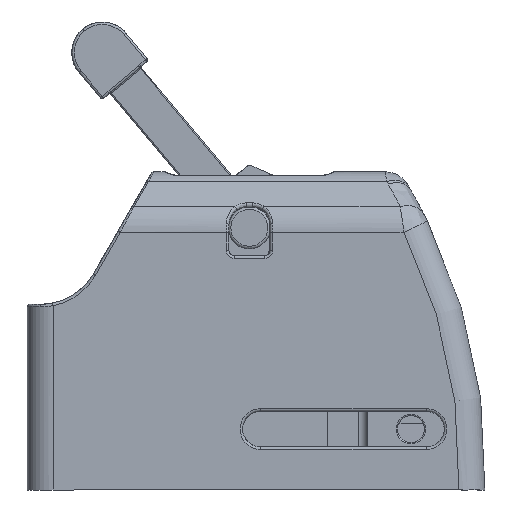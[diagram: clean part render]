
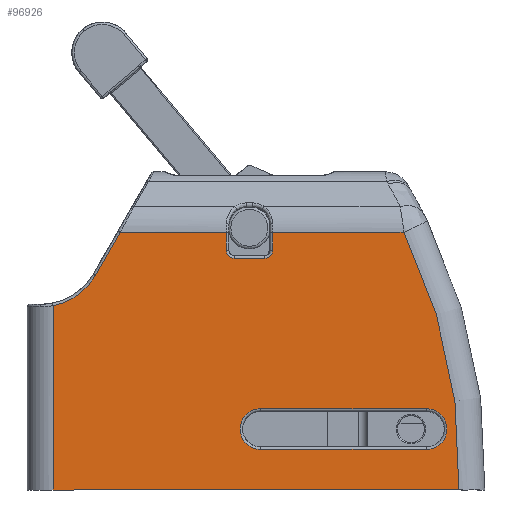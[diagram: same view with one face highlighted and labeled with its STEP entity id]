
A CAD part, left-side view. The second image highlights one B-rep face of the part: STEP entity #96926.
In plain terms, the highlighted planar face has unit normal (-1, 0, 0).
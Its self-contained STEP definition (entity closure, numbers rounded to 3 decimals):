
#5183=FACE_BOUND('',#18355,.T.);
#10724=PLANE('',#102975);
#12639=FACE_OUTER_BOUND('',#18354,.T.);
#18354=EDGE_LOOP('',(#66853,#66854,#66855,#66856,#66857,#66858,#66859,#66860,
#66861,#66862,#66863,#66864));
#18355=EDGE_LOOP('',(#66865,#66866,#66867,#66868));
#24453=LINE('',#128209,#31657);
#24456=LINE('',#128224,#31660);
#24464=LINE('',#128274,#31668);
#24465=LINE('',#128278,#31669);
#24466=LINE('',#128280,#31670);
#24467=LINE('',#128284,#31671);
#24468=LINE('',#128286,#31672);
#24469=LINE('',#128290,#31673);
#24470=LINE('',#128294,#31674);
#24471=LINE('',#128295,#31675);
#31657=VECTOR('',#108685,10.);
#31660=VECTOR('',#108702,10.);
#31668=VECTOR('',#108730,10.);
#31669=VECTOR('',#108733,10.);
#31670=VECTOR('',#108734,10.);
#31671=VECTOR('',#108737,10.);
#31672=VECTOR('',#108738,10.);
#31673=VECTOR('',#108741,10.);
#31674=VECTOR('',#108744,10.);
#31675=VECTOR('',#108745,10.);
#38824=CIRCLE('',#102963,3.925);
#38827=CIRCLE('',#102968,3.925);
#38832=CIRCLE('',#102976,12.);
#38833=CIRCLE('',#102977,103.5);
#38834=CIRCLE('',#102978,1.5);
#38835=CIRCLE('',#102979,1.5);
#40448=VERTEX_POINT('',#128206);
#40449=VERTEX_POINT('',#128208);
#40451=VERTEX_POINT('',#128214);
#40453=VERTEX_POINT('',#128220);
#40465=VERTEX_POINT('',#128272);
#40466=VERTEX_POINT('',#128273);
#40467=VERTEX_POINT('',#128275);
#40468=VERTEX_POINT('',#128277);
#40469=VERTEX_POINT('',#128279);
#40470=VERTEX_POINT('',#128281);
#40471=VERTEX_POINT('',#128283);
#40472=VERTEX_POINT('',#128285);
#40473=VERTEX_POINT('',#128287);
#40474=VERTEX_POINT('',#128289);
#40475=VERTEX_POINT('',#128291);
#40476=VERTEX_POINT('',#128293);
#50762=EDGE_CURVE('',#40448,#40449,#24453,.T.);
#50767=EDGE_CURVE('',#40449,#40451,#38824,.T.);
#50770=EDGE_CURVE('',#40451,#40453,#24456,.T.);
#50772=EDGE_CURVE('',#40453,#40448,#38827,.T.);
#50786=EDGE_CURVE('',#40465,#40466,#24464,.T.);
#50787=EDGE_CURVE('',#40467,#40465,#38832,.T.);
#50788=EDGE_CURVE('',#40468,#40467,#24465,.T.);
#50789=EDGE_CURVE('',#40468,#40469,#24466,.F.);
#50790=EDGE_CURVE('',#40470,#40469,#38833,.T.);
#50791=EDGE_CURVE('',#40470,#40471,#24467,.T.);
#50792=EDGE_CURVE('',#40472,#40471,#24468,.T.);
#50793=EDGE_CURVE('',#40473,#40472,#38834,.T.);
#50794=EDGE_CURVE('',#40474,#40473,#24469,.T.);
#50795=EDGE_CURVE('',#40475,#40474,#38835,.T.);
#50796=EDGE_CURVE('',#40476,#40475,#24470,.T.);
#50797=EDGE_CURVE('',#40476,#40466,#24471,.T.);
#66853=ORIENTED_EDGE('',*,*,#50786,.F.);
#66854=ORIENTED_EDGE('',*,*,#50787,.F.);
#66855=ORIENTED_EDGE('',*,*,#50788,.F.);
#66856=ORIENTED_EDGE('',*,*,#50789,.T.);
#66857=ORIENTED_EDGE('',*,*,#50790,.F.);
#66858=ORIENTED_EDGE('',*,*,#50791,.T.);
#66859=ORIENTED_EDGE('',*,*,#50792,.F.);
#66860=ORIENTED_EDGE('',*,*,#50793,.F.);
#66861=ORIENTED_EDGE('',*,*,#50794,.F.);
#66862=ORIENTED_EDGE('',*,*,#50795,.F.);
#66863=ORIENTED_EDGE('',*,*,#50796,.F.);
#66864=ORIENTED_EDGE('',*,*,#50797,.T.);
#66865=ORIENTED_EDGE('',*,*,#50762,.F.);
#66866=ORIENTED_EDGE('',*,*,#50772,.F.);
#66867=ORIENTED_EDGE('',*,*,#50770,.F.);
#66868=ORIENTED_EDGE('',*,*,#50767,.F.);
#96926=ADVANCED_FACE('',(#12639,#5183),#10724,.F.);
#102963=AXIS2_PLACEMENT_3D('',#128218,#108695,#108696);
#102968=AXIS2_PLACEMENT_3D('',#128227,#108707,#108708);
#102975=AXIS2_PLACEMENT_3D('',#128271,#108728,#108729);
#102976=AXIS2_PLACEMENT_3D('',#128276,#108731,#108732);
#102977=AXIS2_PLACEMENT_3D('',#128282,#108735,#108736);
#102978=AXIS2_PLACEMENT_3D('',#128288,#108739,#108740);
#102979=AXIS2_PLACEMENT_3D('',#128292,#108742,#108743);
#108685=DIRECTION('',(0.,-1.,0.));
#108695=DIRECTION('center_axis',(-1.,0.,0.));
#108696=DIRECTION('ref_axis',(0.,-1.,0.));
#108702=DIRECTION('',(0.,1.,0.));
#108707=DIRECTION('center_axis',(-1.,0.,0.));
#108708=DIRECTION('ref_axis',(0.,1.,0.));
#108728=DIRECTION('center_axis',(1.,0.,0.));
#108729=DIRECTION('ref_axis',(0.,0.,-1.));
#108730=DIRECTION('',(0.,-0.499,0.866));
#108731=DIRECTION('center_axis',(-1.,0.,0.));
#108732=DIRECTION('ref_axis',(0.,-0.583,-0.812));
#108733=DIRECTION('',(0.,0.,1.));
#108734=DIRECTION('',(0.,1.,0.));
#108735=DIRECTION('center_axis',(1.,0.,0.));
#108736=DIRECTION('ref_axis',(0.,-0.976,
0.216));
#108737=DIRECTION('',(0.,1.,0.));
#108738=DIRECTION('',(0.,0.,1.));
#108739=DIRECTION('center_axis',(-1.,0.,0.));
#108740=DIRECTION('ref_axis',(0.,-0.707,-0.707));
#108741=DIRECTION('',(0.,-1.,0.));
#108742=DIRECTION('center_axis',(-1.,0.,0.));
#108743=DIRECTION('ref_axis',(0.,0.707,-0.707));
#108744=DIRECTION('',(0.,0.,-1.));
#108745=DIRECTION('',(0.,1.,0.));
#128206=CARTESIAN_POINT('',(-258.44,-13.233,-12.45));
#128208=CARTESIAN_POINT('',(-258.44,-45.212,-12.45));
#128209=CARTESIAN_POINT('',(-258.44,-12.819,-12.45));
#128214=CARTESIAN_POINT('',(-258.44,-45.212,-4.6));
#128218=CARTESIAN_POINT('Origin',(-258.44,-45.212,-8.525));
#128220=CARTESIAN_POINT('',(-258.44,-13.233,-4.6));
#128224=CARTESIAN_POINT('',(-258.44,-12.819,-4.6));
#128227=CARTESIAN_POINT('Origin',(-258.44,-13.233,-8.525));
#128271=CARTESIAN_POINT('Origin',(-258.44,-12.406,8.812));
#128272=CARTESIAN_POINT('',(-258.44,18.591,21.057));
#128273=CARTESIAN_POINT('',(-258.44,13.797,29.372));
#128274=CARTESIAN_POINT('',(-258.44,11.452,33.44));
#128275=CARTESIAN_POINT('',(-258.44,26.734,15.264));
#128276=CARTESIAN_POINT('Origin',(-258.44,28.987,27.051));
#128277=CARTESIAN_POINT('',(-258.44,26.734,-20.259));
#128278=CARTESIAN_POINT('',(-258.44,26.734,14.575));
#128279=CARTESIAN_POINT('',(-258.44,-51.472,-20.259));
#128280=CARTESIAN_POINT('',(-258.44,-6.203,-20.259));
#128281=CARTESIAN_POINT('',(-258.44,-40.894,29.372));
#128282=CARTESIAN_POINT('Origin',(-258.44,51.954,-16.36));
#128283=CARTESIAN_POINT('',(-258.44,-15.567,29.372));
#128284=CARTESIAN_POINT('',(-258.44,-56.546,29.372));
#128285=CARTESIAN_POINT('',(-258.44,-15.567,25.905));
#128286=CARTESIAN_POINT('',(-258.44,-15.567,16.859));
#128287=CARTESIAN_POINT('',(-258.44,-14.067,24.405));
#128288=CARTESIAN_POINT('Origin',(-258.44,-14.067,25.905));
#128289=CARTESIAN_POINT('',(-258.44,-8.167,24.405));
#128290=CARTESIAN_POINT('',(-258.44,-9.786,24.405));
#128291=CARTESIAN_POINT('',(-258.44,-6.667,25.905));
#128292=CARTESIAN_POINT('Origin',(-258.44,-8.167,25.905));
#128293=CARTESIAN_POINT('',(-258.44,-6.667,29.372));
#128294=CARTESIAN_POINT('',(-258.44,-6.667,19.859));
#128295=CARTESIAN_POINT('',(-258.44,-56.546,29.372));
